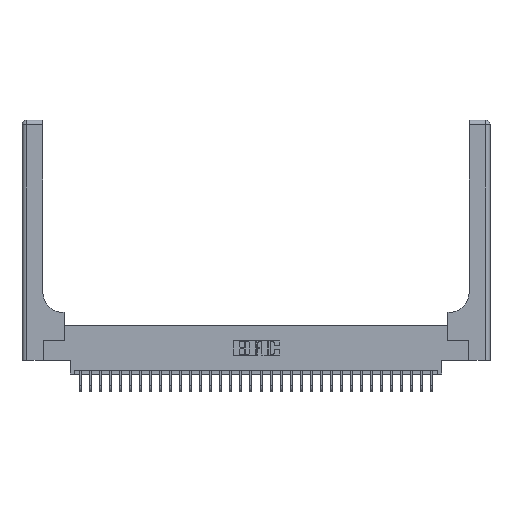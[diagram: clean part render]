
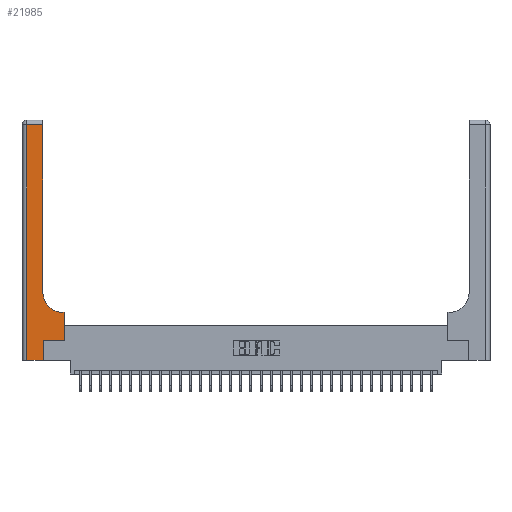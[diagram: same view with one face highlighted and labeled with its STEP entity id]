
A CAD part, top view. The second image highlights one B-rep face of the part: STEP entity #21985.
In plain terms, the highlighted planar face has unit normal (0, 0, 1).
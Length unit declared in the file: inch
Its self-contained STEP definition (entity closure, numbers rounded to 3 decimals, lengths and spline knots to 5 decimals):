
#555 = VERTEX_POINT ( 'NONE', #2702 ) ;
#1083 = CARTESIAN_POINT ( 'NONE',  ( 0.51, 0.85, 0.37 ) ) ;
#1507 = DIRECTION ( 'NONE',  ( 1., 0., 0. ) ) ;
#2702 = CARTESIAN_POINT ( 'NONE',  ( 0.265, 0., 0.37 ) ) ;
#2794 = VECTOR ( 'NONE', #13022, 39.37008 ) ;
#3121 = LINE ( 'NONE', #5071, #4643 ) ;
#3622 = LINE ( 'NONE', #24523, #25628 ) ;
#3687 = EDGE_CURVE ( 'NONE', #26447, #30164, #10832, .T. ) ;
#4080 = AXIS2_PLACEMENT_3D ( 'NONE', #14041, #30878, #11513 ) ;
#4345 = ORIENTED_EDGE ( 'NONE', *, *, #4993, .T. ) ;
#4399 = EDGE_CURVE ( 'NONE', #7518, #12075, #10043, .T. ) ;
#4521 = EDGE_CURVE ( 'NONE', #27842, #4979, #25960, .T. ) ;
#4643 = VECTOR ( 'NONE', #14748, 39.37008 ) ;
#4966 = CARTESIAN_POINT ( 'NONE',  ( 0., 0., 0.37 ) ) ;
#4979 = VERTEX_POINT ( 'NONE', #8326 ) ;
#4993 = EDGE_CURVE ( 'NONE', #17284, #7518, #6573, .T. ) ;
#5071 = CARTESIAN_POINT ( 'NONE',  ( 0.265, 0., 0.37 ) ) ;
#5520 = AXIS2_PLACEMENT_3D ( 'NONE', #1083, #30171, #1507 ) ;
#5553 = EDGE_CURVE ( 'NONE', #4979, #26447, #21749, .T. ) ;
#6239 = VECTOR ( 'NONE', #10361, 39.37008 ) ;
#6400 = CARTESIAN_POINT ( 'NONE',  ( 0.51, 0.6, 0.37 ) ) ;
#6573 = LINE ( 'NONE', #27745, #16445 ) ;
#7352 = CIRCLE ( 'NONE', #5520, 0.25 ) ;
#7518 = VERTEX_POINT ( 'NONE', #29889 ) ;
#7630 = CARTESIAN_POINT ( 'NONE',  ( 0.26, 0.6, 0.37 ) ) ;
#8326 = CARTESIAN_POINT ( 'NONE',  ( 0.26, 2.94, 0.37 ) ) ;
#9016 = VERTEX_POINT ( 'NONE', #23308 ) ;
#9931 = CARTESIAN_POINT ( 'NONE',  ( 0.528, 0.25, 0.37 ) ) ;
#10043 = LINE ( 'NONE', #7630, #6239 ) ;
#10361 = DIRECTION ( 'NONE',  ( -1., 0., 0. ) ) ;
#10832 = LINE ( 'NONE', #23519, #23413 ) ;
#11407 = DIRECTION ( 'NONE',  ( 0., -1., 0. ) ) ;
#11513 = DIRECTION ( 'NONE',  ( -1., 0., 0. ) ) ;
#11710 = ORIENTED_EDGE ( 'NONE', *, *, #17978, .T. ) ;
#11772 = ORIENTED_EDGE ( 'NONE', *, *, #4399, .T. ) ;
#12075 = VERTEX_POINT ( 'NONE', #6400 ) ;
#12893 = DIRECTION ( 'NONE',  ( 0., 1., 0. ) ) ;
#13022 = DIRECTION ( 'NONE',  ( 0., 1., 0. ) ) ;
#14041 = CARTESIAN_POINT ( 'NONE',  ( 0., 3., 0.37 ) ) ;
#14084 = VECTOR ( 'NONE', #23980, 39.37008 ) ;
#14096 = ORIENTED_EDGE ( 'NONE', *, *, #5553, .T. ) ;
#14748 = DIRECTION ( 'NONE',  ( 0., 1., 0. ) ) ;
#15183 = DIRECTION ( 'NONE',  ( -1., 0., 0. ) ) ;
#16445 = VECTOR ( 'NONE', #12893, 39.37008 ) ;
#17284 = VERTEX_POINT ( 'NONE', #9931 ) ;
#17584 = ORIENTED_EDGE ( 'NONE', *, *, #4521, .T. ) ;
#17978 = EDGE_CURVE ( 'NONE', #30164, #555, #24700, .T. ) ;
#17990 = FACE_OUTER_BOUND ( 'NONE', #20563, .T. ) ;
#18943 = PLANE ( 'NONE',  #4080 ) ;
#19519 = ORIENTED_EDGE ( 'NONE', *, *, #30928, .T. ) ;
#20563 = EDGE_LOOP ( 'NONE', ( #17584, #14096, #30008, #11710, #19519, #22127, #4345, #11772, #25241 ) ) ;
#21749 = LINE ( 'NONE', #22416, #26666 ) ;
#21804 = EDGE_CURVE ( 'NONE', #12075, #27842, #7352, .T. ) ;
#21985 = ADVANCED_FACE ( 'NONE', ( #17990 ), #18943, .F. ) ;
#22127 = ORIENTED_EDGE ( 'NONE', *, *, #29731, .T. ) ;
#22416 = CARTESIAN_POINT ( 'NONE',  ( 0., 2.94, 0.37 ) ) ;
#23308 = CARTESIAN_POINT ( 'NONE',  ( 0.265, 0.25, 0.37 ) ) ;
#23413 = VECTOR ( 'NONE', #11407, 39.37008 ) ;
#23519 = CARTESIAN_POINT ( 'NONE',  ( 0.06, 3., 0.37 ) ) ;
#23980 = DIRECTION ( 'NONE',  ( 1., 0., 0. ) ) ;
#24523 = CARTESIAN_POINT ( 'NONE',  ( 0.265, 0.25, 0.37 ) ) ;
#24700 = LINE ( 'NONE', #4966, #14084 ) ;
#25168 = CARTESIAN_POINT ( 'NONE',  ( 0.06, 2.94, 0.37 ) ) ;
#25241 = ORIENTED_EDGE ( 'NONE', *, *, #21804, .T. ) ;
#25628 = VECTOR ( 'NONE', #29117, 39.37008 ) ;
#25960 = LINE ( 'NONE', #29801, #2794 ) ;
#26447 = VERTEX_POINT ( 'NONE', #25168 ) ;
#26666 = VECTOR ( 'NONE', #15183, 39.37008 ) ;
#27745 = CARTESIAN_POINT ( 'NONE',  ( 0.528, 0.25, 0.37 ) ) ;
#27842 = VERTEX_POINT ( 'NONE', #28598 ) ;
#28598 = CARTESIAN_POINT ( 'NONE',  ( 0.26, 0.85, 0.37 ) ) ;
#29117 = DIRECTION ( 'NONE',  ( 1., 0., 0. ) ) ;
#29731 = EDGE_CURVE ( 'NONE', #9016, #17284, #3622, .T. ) ;
#29801 = CARTESIAN_POINT ( 'NONE',  ( 0.26, 3., 0.37 ) ) ;
#29889 = CARTESIAN_POINT ( 'NONE',  ( 0.528, 0.6, 0.37 ) ) ;
#30008 = ORIENTED_EDGE ( 'NONE', *, *, #3687, .T. ) ;
#30164 = VERTEX_POINT ( 'NONE', #30812 ) ;
#30171 = DIRECTION ( 'NONE',  ( 0., 0., -1. ) ) ;
#30812 = CARTESIAN_POINT ( 'NONE',  ( 0.06, 0., 0.37 ) ) ;
#30878 = DIRECTION ( 'NONE',  ( 0., 0., -1. ) ) ;
#30928 = EDGE_CURVE ( 'NONE', #555, #9016, #3121, .T. ) ;
